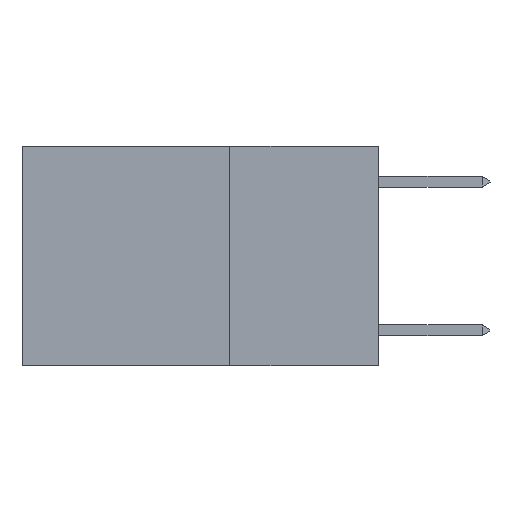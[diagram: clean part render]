
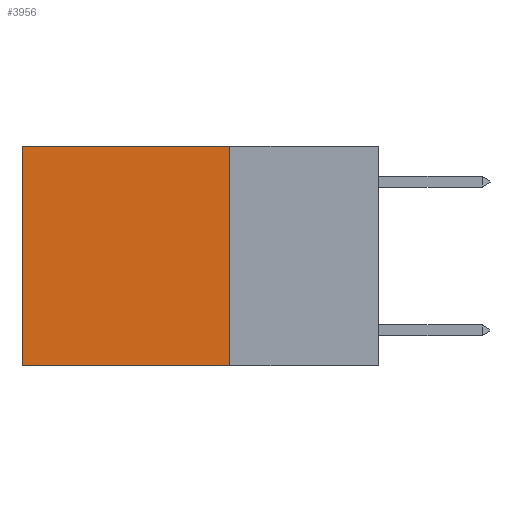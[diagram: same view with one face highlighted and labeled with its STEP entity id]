
A CAD part, left-side view. The second image highlights one B-rep face of the part: STEP entity #3956.
In plain terms, the highlighted planar face has unit normal (-1, 0, 0).
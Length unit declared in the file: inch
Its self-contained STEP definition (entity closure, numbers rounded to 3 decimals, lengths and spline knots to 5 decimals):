
#100 = VERTEX_POINT ( 'NONE', #3773 ) ;
#304 = EDGE_CURVE ( 'NONE', #100, #1196, #2839, .T. ) ;
#573 = DIRECTION ( 'NONE',  ( 0., 1., 0. ) ) ;
#674 = EDGE_LOOP ( 'NONE', ( #9257, #2476, #4736, #4185 ) ) ;
#1003 = VECTOR ( 'NONE', #573, 39.37008 ) ;
#1196 = VERTEX_POINT ( 'NONE', #8716 ) ;
#1624 = CARTESIAN_POINT ( 'NONE',  ( 0.2625, 0.25, -0.37 ) ) ;
#1841 = CARTESIAN_POINT ( 'NONE',  ( 0.2625, 0.6, 0. ) ) ;
#1853 = EDGE_CURVE ( 'NONE', #8995, #3226, #5648, .T. ) ;
#2476 = ORIENTED_EDGE ( 'NONE', *, *, #1853, .F. ) ;
#2639 = DIRECTION ( 'NONE',  ( 0., 0., -1. ) ) ;
#2830 = CARTESIAN_POINT ( 'NONE',  ( 0.2625, 0.25, 0. ) ) ;
#2839 = LINE ( 'NONE', #7480, #1003 ) ;
#2880 = CARTESIAN_POINT ( 'NONE',  ( 0.2625, 0.25, 0. ) ) ;
#3211 = DIRECTION ( 'NONE',  ( 0., 1., 0. ) ) ;
#3226 = VERTEX_POINT ( 'NONE', #5755 ) ;
#3646 = PLANE ( 'NONE',  #6190 ) ;
#3663 = DIRECTION ( 'NONE',  ( 0., 0., -1. ) ) ;
#3773 = CARTESIAN_POINT ( 'NONE',  ( 0.2625, 0.25, 0. ) ) ;
#3956 = ADVANCED_FACE ( 'NONE', ( #4788 ), #3646, .F. ) ;
#4185 = ORIENTED_EDGE ( 'NONE', *, *, #304, .T. ) ;
#4477 = DIRECTION ( 'NONE',  ( 0., 0., -1. ) ) ;
#4569 = EDGE_CURVE ( 'NONE', #100, #8995, #6221, .T. ) ;
#4577 = LINE ( 'NONE', #1841, #8478 ) ;
#4736 = ORIENTED_EDGE ( 'NONE', *, *, #4569, .F. ) ;
#4788 = FACE_OUTER_BOUND ( 'NONE', #674, .T. ) ;
#5648 = LINE ( 'NONE', #1624, #7510 ) ;
#5755 = CARTESIAN_POINT ( 'NONE',  ( 0.2625, 0.6, -0.37 ) ) ;
#6190 = AXIS2_PLACEMENT_3D ( 'NONE', #2830, #9132, #4477 ) ;
#6221 = LINE ( 'NONE', #2880, #8328 ) ;
#6478 = CARTESIAN_POINT ( 'NONE',  ( 0.2625, 0.25, -0.37 ) ) ;
#7480 = CARTESIAN_POINT ( 'NONE',  ( 0.2625, 0.25, 0. ) ) ;
#7510 = VECTOR ( 'NONE', #3211, 39.37008 ) ;
#8328 = VECTOR ( 'NONE', #3663, 39.37008 ) ;
#8478 = VECTOR ( 'NONE', #2639, 39.37008 ) ;
#8514 = EDGE_CURVE ( 'NONE', #1196, #3226, #4577, .T. ) ;
#8716 = CARTESIAN_POINT ( 'NONE',  ( 0.2625, 0.6, 0. ) ) ;
#8995 = VERTEX_POINT ( 'NONE', #6478 ) ;
#9132 = DIRECTION ( 'NONE',  ( 1., 0., 0. ) ) ;
#9257 = ORIENTED_EDGE ( 'NONE', *, *, #8514, .T. ) ;
